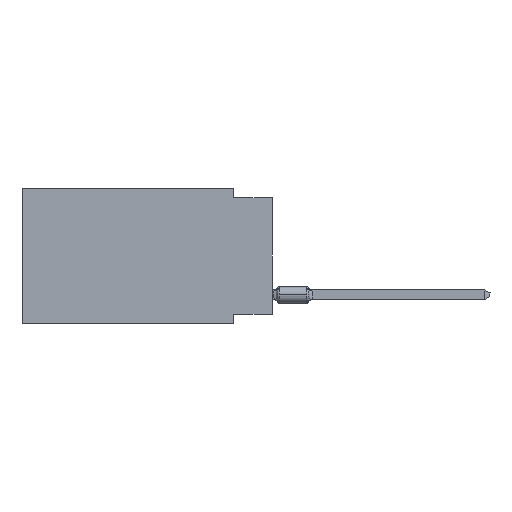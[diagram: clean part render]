
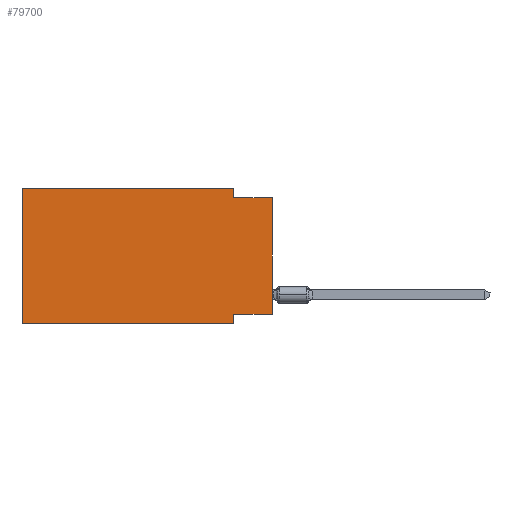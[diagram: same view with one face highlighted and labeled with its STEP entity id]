
A CAD part, left-side view. The second image highlights one B-rep face of the part: STEP entity #79700.
In plain terms, the highlighted planar face has unit normal (-1, 0, 0).
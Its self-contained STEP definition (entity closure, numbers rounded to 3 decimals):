
#493 = ORIENTED_EDGE ( 'NONE', *, *, #7767, .F. ) ;
#1377 = DIRECTION ( 'NONE',  ( 0., -1., 0. ) ) ;
#2561 = ORIENTED_EDGE ( 'NONE', *, *, #71481, .F. ) ;
#3753 = EDGE_CURVE ( 'NONE', #66187, #71616, #59496, .T. ) ;
#4704 = DIRECTION ( 'NONE',  ( 0., 0., 1. ) ) ;
#6930 = CARTESIAN_POINT ( 'NONE',  ( 0., 16.383, 0. ) ) ;
#7767 = EDGE_CURVE ( 'NONE', #66187, #65155, #17514, .T. ) ;
#9093 = VERTEX_POINT ( 'NONE', #29040 ) ;
#9281 = VECTOR ( 'NONE', #1377, 1000. ) ;
#13130 = ORIENTED_EDGE ( 'NONE', *, *, #15686, .F. ) ;
#13211 = VECTOR ( 'NONE', #70628, 1000. ) ;
#13532 = LINE ( 'NONE', #80173, #81044 ) ;
#15686 = EDGE_CURVE ( 'NONE', #44748, #71616, #13532, .T. ) ;
#17514 = LINE ( 'NONE', #68793, #44376 ) ;
#19348 = LINE ( 'NONE', #50962, #13211 ) ;
#19862 = LINE ( 'NONE', #45492, #27243 ) ;
#19993 = CARTESIAN_POINT ( 'NONE',  ( 0., 16.383, 0. ) ) ;
#24230 = EDGE_LOOP ( 'NONE', ( #37635, #66206, #2561, #53713, #493, #30974, #13130, #42928 ) ) ;
#27243 = VECTOR ( 'NONE', #66425, 1000. ) ;
#27639 = CARTESIAN_POINT ( 'NONE',  ( 0., 2.54, -0.635 ) ) ;
#29040 = CARTESIAN_POINT ( 'NONE',  ( 0., 0., -0.635 ) ) ;
#30974 = ORIENTED_EDGE ( 'NONE', *, *, #3753, .T. ) ;
#32217 = CARTESIAN_POINT ( 'NONE',  ( 0., 16.383, -8.89 ) ) ;
#32639 = DIRECTION ( 'NONE',  ( 0., 0., -1. ) ) ;
#33589 = DIRECTION ( 'NONE',  ( 0., 0., -1. ) ) ;
#33645 = DIRECTION ( 'NONE',  ( 1., 0., 0. ) ) ;
#34669 = DIRECTION ( 'NONE',  ( 0., -1., 0. ) ) ;
#36715 = CARTESIAN_POINT ( 'NONE',  ( 0., 16.383, 0. ) ) ;
#37635 = ORIENTED_EDGE ( 'NONE', *, *, #73599, .T. ) ;
#39045 = LINE ( 'NONE', #65120, #46623 ) ;
#40029 = VECTOR ( 'NONE', #75468, 1000. ) ;
#40476 = FACE_OUTER_BOUND ( 'NONE', #24230, .T. ) ;
#42928 = ORIENTED_EDGE ( 'NONE', *, *, #54488, .F. ) ;
#44158 = CARTESIAN_POINT ( 'NONE',  ( 0., 2.54, 0. ) ) ;
#44376 = VECTOR ( 'NONE', #4704, 1000. ) ;
#44748 = VERTEX_POINT ( 'NONE', #50336 ) ;
#45492 = CARTESIAN_POINT ( 'NONE',  ( 0., 0., -8.255 ) ) ;
#46623 = VECTOR ( 'NONE', #32639, 1000. ) ;
#46894 = DIRECTION ( 'NONE',  ( 0., 0., -1. ) ) ;
#50336 = CARTESIAN_POINT ( 'NONE',  ( 0., 2.54, -8.255 ) ) ;
#50962 = CARTESIAN_POINT ( 'NONE',  ( 0., 0., -0.635 ) ) ;
#52229 = LINE ( 'NONE', #6930, #9281 ) ;
#53713 = ORIENTED_EDGE ( 'NONE', *, *, #67886, .F. ) ;
#54139 = CARTESIAN_POINT ( 'NONE',  ( 0., 0., 0. ) ) ;
#54488 = EDGE_CURVE ( 'NONE', #77273, #44748, #19862, .T. ) ;
#55873 = VERTEX_POINT ( 'NONE', #27639 ) ;
#59496 = LINE ( 'NONE', #79165, #71047 ) ;
#59605 = CARTESIAN_POINT ( 'NONE',  ( 0., 0., -8.255 ) ) ;
#65120 = CARTESIAN_POINT ( 'NONE',  ( 0., 2.54, 0. ) ) ;
#65155 = VERTEX_POINT ( 'NONE', #36715 ) ;
#66187 = VERTEX_POINT ( 'NONE', #32217 ) ;
#66206 = ORIENTED_EDGE ( 'NONE', *, *, #77553, .F. ) ;
#66425 = DIRECTION ( 'NONE',  ( 0., 1., 0. ) ) ;
#66977 = LINE ( 'NONE', #54139, #40029 ) ;
#67886 = EDGE_CURVE ( 'NONE', #65155, #69665, #52229, .T. ) ;
#68793 = CARTESIAN_POINT ( 'NONE',  ( 0., 16.383, 0. ) ) ;
#69665 = VERTEX_POINT ( 'NONE', #44158 ) ;
#70628 = DIRECTION ( 'NONE',  ( 0., -1., 0. ) ) ;
#71047 = VECTOR ( 'NONE', #34669, 1000. ) ;
#71481 = EDGE_CURVE ( 'NONE', #69665, #55873, #39045, .T. ) ;
#71616 = VERTEX_POINT ( 'NONE', #76044 ) ;
#72850 = AXIS2_PLACEMENT_3D ( 'NONE', #19993, #33645, #46894 ) ;
#73394 = PLANE ( 'NONE',  #72850 ) ;
#73599 = EDGE_CURVE ( 'NONE', #77273, #9093, #66977, .T. ) ;
#75468 = DIRECTION ( 'NONE',  ( 0., 0., 1. ) ) ;
#76044 = CARTESIAN_POINT ( 'NONE',  ( 0., 2.54, -8.89 ) ) ;
#77273 = VERTEX_POINT ( 'NONE', #59605 ) ;
#77553 = EDGE_CURVE ( 'NONE', #55873, #9093, #19348, .T. ) ;
#79165 = CARTESIAN_POINT ( 'NONE',  ( 0., 16.383, -8.89 ) ) ;
#79700 = ADVANCED_FACE ( 'NONE', ( #40476 ), #73394, .F. ) ;
#80173 = CARTESIAN_POINT ( 'NONE',  ( 0., 2.54, -8.89 ) ) ;
#81044 = VECTOR ( 'NONE', #33589, 1000. ) ;
